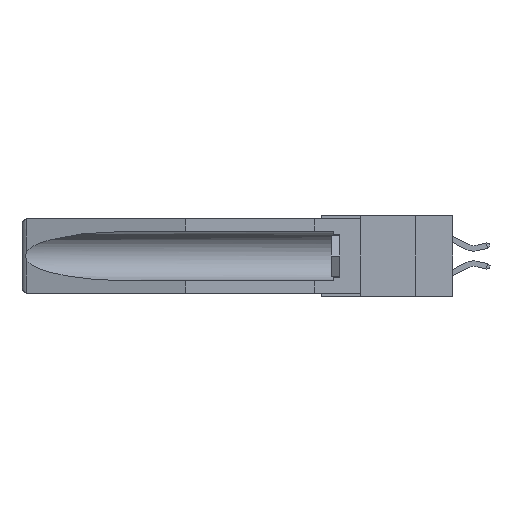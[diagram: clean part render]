
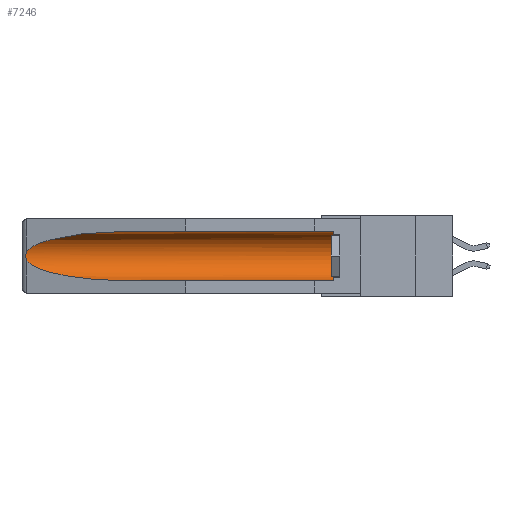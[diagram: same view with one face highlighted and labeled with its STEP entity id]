
A CAD part, left-side view. The second image highlights one B-rep face of the part: STEP entity #7246.
In plain terms, the highlighted cylindrical face has radius 2.857 mm (diameter 5.715 mm), a partial arc.
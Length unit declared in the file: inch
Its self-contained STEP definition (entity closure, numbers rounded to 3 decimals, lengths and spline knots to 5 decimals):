
#276 = VECTOR ( 'NONE', #13680, 39.37008 ) ;
#362 = CARTESIAN_POINT ( 'NONE',  ( 0.21114, 1.30732, -0.059 ) ) ;
#631 = VERTEX_POINT ( 'NONE', #4887 ) ;
#1224 = DIRECTION ( 'NONE',  ( 0., 0., 1. ) ) ;
#1580 = EDGE_CURVE ( 'NONE', #15072, #18743, #18164, .T. ) ;
#1719 = B_SPLINE_CURVE_WITH_KNOTS ( 'NONE', 3,
 ( #12419, #7796, #4773, #17517, #1723, #16886, #3285, #3082, #3017, #15267 ),
 .UNSPECIFIED., .F., .F.,
 ( 4, 2, 2, 2, 4 ),
 ( 0., 0.00029, 0.00058, 0.00087, 0.00117 ),
 .UNSPECIFIED. ) ;
#1722 = EDGE_CURVE ( 'NONE', #631, #15127, #4075, .T. ) ;
#1723 = CARTESIAN_POINT ( 'NONE',  ( 0.2675, 1.53308, -0.16763 ) ) ;
#1814 = VERTEX_POINT ( 'NONE', #7079 ) ;
#2152 = CARTESIAN_POINT ( 'NONE',  ( 0.155, 1.07973, -0.284 ) ) ;
#2702 = ORIENTED_EDGE ( 'NONE', *, *, #9040, .F. ) ;
#2822 = ORIENTED_EDGE ( 'NONE', *, *, #8758, .T. ) ;
#2855 = CARTESIAN_POINT ( 'NONE',  ( 0.26537, 1.52718, -0.14972 ) ) ;
#3017 = CARTESIAN_POINT ( 'NONE',  ( 0.26597, 1.5296, -0.19026 ) ) ;
#3082 = CARTESIAN_POINT ( 'NONE',  ( 0.26655, 1.53094, -0.18657 ) ) ;
#3174 = CIRCLE ( 'NONE', #16988, 0.1125 ) ;
#3285 = CARTESIAN_POINT ( 'NONE',  ( 0.2673, 1.53269, -0.17917 ) ) ;
#3506 = ORIENTED_EDGE ( 'NONE', *, *, #18278, .T. ) ;
#3724 = CARTESIAN_POINT ( 'NONE',  ( 0.155, 1.07973, -0.059 ) ) ;
#4075 =( BOUNDED_CURVE ( )  B_SPLINE_CURVE ( 3, ( #8383, #5518, #11559, #2152 ),
 .UNSPECIFIED., .F., .F. ) 
 B_SPLINE_CURVE_WITH_KNOTS ( ( 4, 4 ),
 ( 0.1948, 1.5708 ),
 .UNSPECIFIED. ) 
 CURVE ( )  GEOMETRIC_REPRESENTATION_ITEM ( )  RATIONAL_B_SPLINE_CURVE ( ( 1., 0.848, 0.848, 1. ) ) 
 REPRESENTATION_ITEM ( '' )  );
#4394 = LINE ( 'NONE', #10649, #276 ) ;
#4773 = CARTESIAN_POINT ( 'NONE',  ( 0.26654, 1.53092, -0.15636 ) ) ;
#4887 = CARTESIAN_POINT ( 'NONE',  ( 0.26537, 1.52718, -0.19328 ) ) ;
#4915 = CYLINDRICAL_SURFACE ( 'NONE', #17590, 0.1125 ) ;
#5341 = DIRECTION ( 'NONE',  ( 0., 0., 1. ) ) ;
#5518 = CARTESIAN_POINT ( 'NONE',  ( 0.25451, 1.48313, -0.24835 ) ) ;
#5628 = FACE_OUTER_BOUND ( 'NONE', #5719, .T. ) ;
#5719 = EDGE_LOOP ( 'NONE', ( #17074, #3506, #6649, #2702, #2822, #12073 ) ) ;
#6429 = CARTESIAN_POINT ( 'NONE',  ( 0.155, -0.30754, -0.059 ) ) ;
#6649 = ORIENTED_EDGE ( 'NONE', *, *, #1722, .T. ) ;
#6772 = EDGE_CURVE ( 'NONE', #18743, #16864, #14505, .T. ) ;
#7079 = CARTESIAN_POINT ( 'NONE',  ( 0.155, 0.126, -0.284 ) ) ;
#7246 = ADVANCED_FACE ( 'NONE', ( #5628 ), #4915, .F. ) ;
#7796 = CARTESIAN_POINT ( 'NONE',  ( 0.26597, 1.52961, -0.15275 ) ) ;
#8383 = CARTESIAN_POINT ( 'NONE',  ( 0.26537, 1.52718, -0.19328 ) ) ;
#8592 = DIRECTION ( 'NONE',  ( 0., -1., 0. ) ) ;
#8758 = EDGE_CURVE ( 'NONE', #1814, #15072, #3174, .T. ) ;
#8782 = DIRECTION ( 'NONE',  ( 0., 1., 0. ) ) ;
#9027 = CARTESIAN_POINT ( 'NONE',  ( 0.155, 1.07973, -0.284 ) ) ;
#9040 = EDGE_CURVE ( 'NONE', #1814, #15127, #4394, .T. ) ;
#10242 = CARTESIAN_POINT ( 'NONE',  ( 0.155, 0.126, -0.059 ) ) ;
#10649 = CARTESIAN_POINT ( 'NONE',  ( 0.155, -0.30754, -0.284 ) ) ;
#10879 = CARTESIAN_POINT ( 'NONE',  ( 0.26537, 1.52718, -0.14972 ) ) ;
#10946 = VECTOR ( 'NONE', #17114, 39.37008 ) ;
#11502 = CARTESIAN_POINT ( 'NONE',  ( 0.155, 0.126, -0.1715 ) ) ;
#11559 = CARTESIAN_POINT ( 'NONE',  ( 0.21114, 1.30732, -0.284 ) ) ;
#12073 = ORIENTED_EDGE ( 'NONE', *, *, #1580, .T. ) ;
#12419 = CARTESIAN_POINT ( 'NONE',  ( 0.26537, 1.52718, -0.14972 ) ) ;
#12613 = CARTESIAN_POINT ( 'NONE',  ( 0.155, 1.07973, -0.059 ) ) ;
#13680 = DIRECTION ( 'NONE',  ( 0., 1., 0. ) ) ;
#14505 =( BOUNDED_CURVE ( )  B_SPLINE_CURVE ( 3, ( #12613, #362, #18631, #10879 ),
 .UNSPECIFIED., .F., .F. ) 
 B_SPLINE_CURVE_WITH_KNOTS ( ( 4, 4 ),
 ( 4.71239, 6.08839 ),
 .UNSPECIFIED. ) 
 CURVE ( )  GEOMETRIC_REPRESENTATION_ITEM ( )  RATIONAL_B_SPLINE_CURVE ( ( 1., 0.848, 0.848, 1. ) ) 
 REPRESENTATION_ITEM ( '' )  );
#15072 = VERTEX_POINT ( 'NONE', #10242 ) ;
#15090 = CARTESIAN_POINT ( 'NONE',  ( 0.155, -0.30754, -0.1715 ) ) ;
#15127 = VERTEX_POINT ( 'NONE', #9027 ) ;
#15267 = CARTESIAN_POINT ( 'NONE',  ( 0.26537, 1.52718, -0.19328 ) ) ;
#16864 = VERTEX_POINT ( 'NONE', #2855 ) ;
#16886 = CARTESIAN_POINT ( 'NONE',  ( 0.2675, 1.53308, -0.17534 ) ) ;
#16988 = AXIS2_PLACEMENT_3D ( 'NONE', #11502, #8592, #5341 ) ;
#17074 = ORIENTED_EDGE ( 'NONE', *, *, #6772, .T. ) ;
#17114 = DIRECTION ( 'NONE',  ( 0., 1., 0. ) ) ;
#17517 = CARTESIAN_POINT ( 'NONE',  ( 0.2673, 1.5327, -0.16383 ) ) ;
#17590 = AXIS2_PLACEMENT_3D ( 'NONE', #15090, #8782, #1224 ) ;
#18164 = LINE ( 'NONE', #6429, #10946 ) ;
#18278 = EDGE_CURVE ( 'NONE', #16864, #631, #1719, .T. ) ;
#18631 = CARTESIAN_POINT ( 'NONE',  ( 0.25451, 1.48313, -0.09465 ) ) ;
#18743 = VERTEX_POINT ( 'NONE', #3724 ) ;
